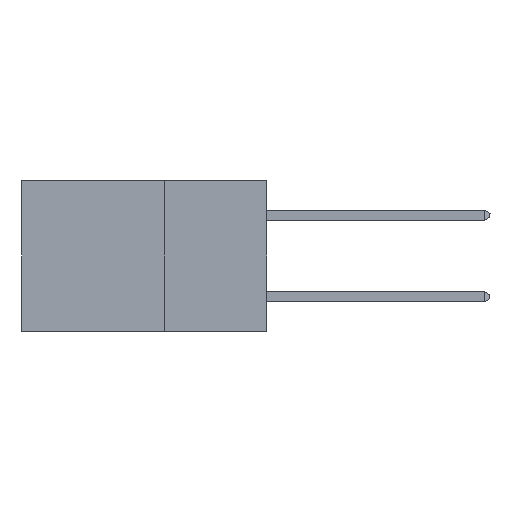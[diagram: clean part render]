
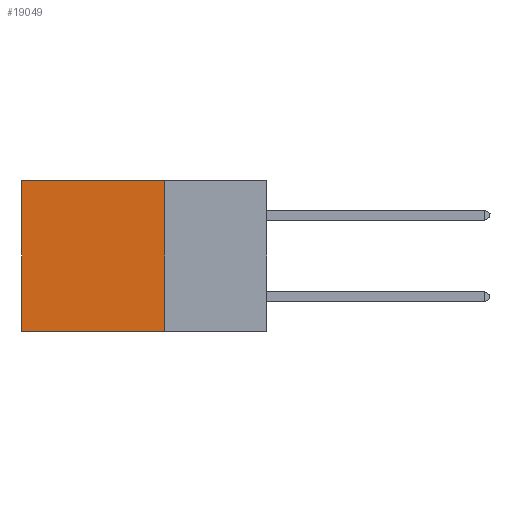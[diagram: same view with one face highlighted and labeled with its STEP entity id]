
A CAD part, left-side view. The second image highlights one B-rep face of the part: STEP entity #19049.
In plain terms, the highlighted planar face has unit normal (-1, 0, 0).
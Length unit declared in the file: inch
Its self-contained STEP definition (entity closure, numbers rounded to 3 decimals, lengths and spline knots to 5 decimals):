
#320 = ORIENTED_EDGE ( 'NONE', *, *, #17165, .F. ) ;
#787 = VECTOR ( 'NONE', #18317, 39.37008 ) ;
#932 = VERTEX_POINT ( 'NONE', #15827 ) ;
#955 = VERTEX_POINT ( 'NONE', #11857 ) ;
#1226 = DIRECTION ( 'NONE',  ( 1., 0., 0. ) ) ;
#1760 = EDGE_CURVE ( 'NONE', #932, #7030, #14193, .T. ) ;
#1835 = CARTESIAN_POINT ( 'NONE',  ( 0.2875, 0.6, -0.37 ) ) ;
#2221 = EDGE_LOOP ( 'NONE', ( #4077, #320, #12699, #16865 ) ) ;
#2351 = LINE ( 'NONE', #12336, #17243 ) ;
#4077 = ORIENTED_EDGE ( 'NONE', *, *, #1760, .T. ) ;
#4705 = AXIS2_PLACEMENT_3D ( 'NONE', #10330, #1226, #11822 ) ;
#7030 = VERTEX_POINT ( 'NONE', #1835 ) ;
#7345 = CARTESIAN_POINT ( 'NONE',  ( 0.2875, 0.25, -0.37 ) ) ;
#7564 = CARTESIAN_POINT ( 'NONE',  ( 0.2875, 0.25, -0.37 ) ) ;
#9364 = FACE_OUTER_BOUND ( 'NONE', #2221, .T. ) ;
#9387 = DIRECTION ( 'NONE',  ( 0., 0., -1. ) ) ;
#9650 = CARTESIAN_POINT ( 'NONE',  ( 0.2875, 0.6, 0. ) ) ;
#10281 = VECTOR ( 'NONE', #14991, 39.37008 ) ;
#10330 = CARTESIAN_POINT ( 'NONE',  ( 0.2875, 0.25, 0. ) ) ;
#11040 = VERTEX_POINT ( 'NONE', #7564 ) ;
#11053 = VECTOR ( 'NONE', #18971, 39.37008 ) ;
#11523 = LINE ( 'NONE', #7345, #11053 ) ;
#11822 = DIRECTION ( 'NONE',  ( 0., 0., -1. ) ) ;
#11857 = CARTESIAN_POINT ( 'NONE',  ( 0.2875, 0.25, 0. ) ) ;
#12336 = CARTESIAN_POINT ( 'NONE',  ( 0.2875, 0.25, 0. ) ) ;
#12699 = ORIENTED_EDGE ( 'NONE', *, *, #16172, .F. ) ;
#12835 = LINE ( 'NONE', #16859, #787 ) ;
#13232 = PLANE ( 'NONE',  #4705 ) ;
#14193 = LINE ( 'NONE', #9650, #10281 ) ;
#14991 = DIRECTION ( 'NONE',  ( 0., 0., -1. ) ) ;
#15827 = CARTESIAN_POINT ( 'NONE',  ( 0.2875, 0.6, 0. ) ) ;
#16172 = EDGE_CURVE ( 'NONE', #955, #11040, #2351, .T. ) ;
#16859 = CARTESIAN_POINT ( 'NONE',  ( 0.2875, 0.25, 0. ) ) ;
#16865 = ORIENTED_EDGE ( 'NONE', *, *, #18655, .T. ) ;
#17165 = EDGE_CURVE ( 'NONE', #11040, #7030, #11523, .T. ) ;
#17243 = VECTOR ( 'NONE', #9387, 39.37008 ) ;
#18317 = DIRECTION ( 'NONE',  ( 0., 1., 0. ) ) ;
#18655 = EDGE_CURVE ( 'NONE', #955, #932, #12835, .T. ) ;
#18971 = DIRECTION ( 'NONE',  ( 0., 1., 0. ) ) ;
#19049 = ADVANCED_FACE ( 'NONE', ( #9364 ), #13232, .F. ) ;
